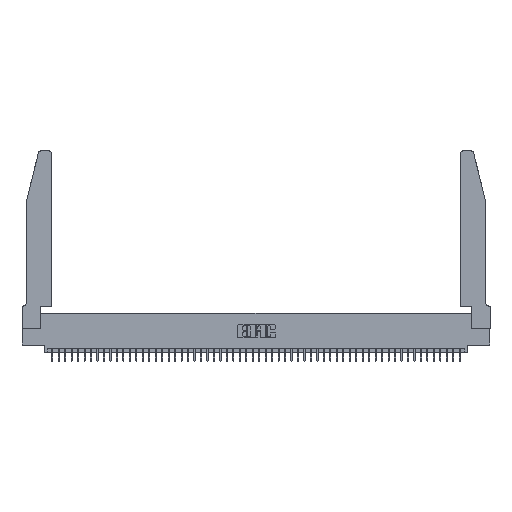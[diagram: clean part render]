
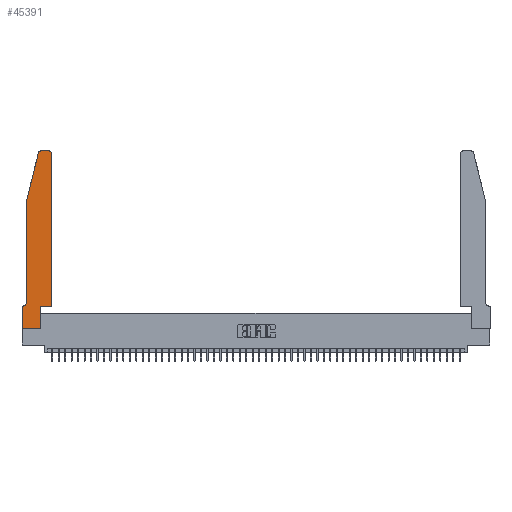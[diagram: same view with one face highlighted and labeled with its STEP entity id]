
A CAD part, top view. The second image highlights one B-rep face of the part: STEP entity #45391.
In plain terms, the highlighted planar face has unit normal (0, 0, 1).
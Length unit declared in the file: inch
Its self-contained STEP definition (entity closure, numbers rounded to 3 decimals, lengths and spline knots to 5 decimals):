
#386 = CARTESIAN_POINT ( 'NONE',  ( 0.284, 2.75, 0.37 ) ) ;
#459 = LINE ( 'NONE', #8402, #41374 ) ;
#460 = ORIENTED_EDGE ( 'NONE', *, *, #44067, .T. ) ;
#944 = CARTESIAN_POINT ( 'NONE',  ( 0.4505, 0.35, 0.37 ) ) ;
#1328 = EDGE_CURVE ( 'NONE', #50639, #6723, #50533, .T. ) ;
#1587 = VERTEX_POINT ( 'NONE', #25113 ) ;
#2338 = AXIS2_PLACEMENT_3D ( 'NONE', #5285, #25363, #17427 ) ;
#2593 = CARTESIAN_POINT ( 'NONE',  ( 0.4205, 2.75, 0.37 ) ) ;
#2871 = LINE ( 'NONE', #31416, #31472 ) ;
#3505 = AXIS2_PLACEMENT_3D ( 'NONE', #18943, #39812, #23174 ) ;
#3706 = ORIENTED_EDGE ( 'NONE', *, *, #1328, .T. ) ;
#4463 = CARTESIAN_POINT ( 'NONE',  ( 0.0055, 0.35, 0.37 ) ) ;
#5285 = CARTESIAN_POINT ( 'NONE',  ( 0.0055, 0.42, 0.37 ) ) ;
#5765 = EDGE_CURVE ( 'NONE', #28128, #6546, #41773, .T. ) ;
#5894 = ORIENTED_EDGE ( 'NONE', *, *, #25072, .T. ) ;
#6160 = AXIS2_PLACEMENT_3D ( 'NONE', #21103, #44902, #8698 ) ;
#6546 = VERTEX_POINT ( 'NONE', #24701 ) ;
#6723 = VERTEX_POINT ( 'NONE', #49540 ) ;
#6933 = ORIENTED_EDGE ( 'NONE', *, *, #7925, .T. ) ;
#7180 = EDGE_CURVE ( 'NONE', #6723, #8515, #17484, .T. ) ;
#7925 = EDGE_CURVE ( 'NONE', #8515, #28151, #41663, .T. ) ;
#8402 = CARTESIAN_POINT ( 'NONE',  ( 0.0755, 2., 0.37 ) ) ;
#8515 = VERTEX_POINT ( 'NONE', #18974 ) ;
#8698 = DIRECTION ( 'NONE',  ( 1., 0., 0. ) ) ;
#10271 = VECTOR ( 'NONE', #13387, 39.37008 ) ;
#11066 = LINE ( 'NONE', #18715, #19585 ) ;
#11080 = DIRECTION ( 'NONE',  ( -1., 0., 0. ) ) ;
#11160 = CARTESIAN_POINT ( 'NONE',  ( 0.0755, 0.42, 0.37 ) ) ;
#12344 = ORIENTED_EDGE ( 'NONE', *, *, #20490, .T. ) ;
#12481 = VECTOR ( 'NONE', #25418, 39.37008 ) ;
#12670 = PLANE ( 'NONE',  #6160 ) ;
#13387 = DIRECTION ( 'NONE',  ( 0., 1., 0. ) ) ;
#14039 = VECTOR ( 'NONE', #21319, 39.37008 ) ;
#14208 = CARTESIAN_POINT ( 'NONE',  ( 0.4505, 0.35, 0.37 ) ) ;
#14576 = DIRECTION ( 'NONE',  ( 1., 0., 0. ) ) ;
#15441 = VERTEX_POINT ( 'NONE', #386 ) ;
#17427 = DIRECTION ( 'NONE',  ( -1., 0., 0. ) ) ;
#17484 = LINE ( 'NONE', #29376, #12481 ) ;
#17785 = VERTEX_POINT ( 'NONE', #25896 ) ;
#18014 = CARTESIAN_POINT ( 'NONE',  ( 0., 0., 0.37 ) ) ;
#18715 = CARTESIAN_POINT ( 'NONE',  ( 0., 0., 0.37 ) ) ;
#18902 = CARTESIAN_POINT ( 'NONE',  ( 0., 0., 0.37 ) ) ;
#18943 = CARTESIAN_POINT ( 'NONE',  ( 0.284, 2.72, 0.37 ) ) ;
#18963 = LINE ( 'NONE', #35858, #27461 ) ;
#18974 = CARTESIAN_POINT ( 'NONE',  ( 0.2865, 0.35, 0.37 ) ) ;
#19585 = VECTOR ( 'NONE', #30608, 39.37008 ) ;
#20490 = EDGE_CURVE ( 'NONE', #37545, #31872, #459, .T. ) ;
#20561 = DIRECTION ( 'NONE',  ( 0., -1., 0. ) ) ;
#21103 = CARTESIAN_POINT ( 'NONE',  ( 0., 0.35, 0.37 ) ) ;
#21319 = DIRECTION ( 'NONE',  ( 1., 0., 0. ) ) ;
#22026 = EDGE_CURVE ( 'NONE', #15441, #1587, #45722, .T. ) ;
#23174 = DIRECTION ( 'NONE',  ( 1., 0., 0. ) ) ;
#23194 = DIRECTION ( 'NONE',  ( -0.239, -0.971, 0. ) ) ;
#24701 = CARTESIAN_POINT ( 'NONE',  ( 0., 0.35, 0.37 ) ) ;
#24888 = ORIENTED_EDGE ( 'NONE', *, *, #36820, .T. ) ;
#25072 = EDGE_CURVE ( 'NONE', #17785, #40887, #40025, .T. ) ;
#25113 = CARTESIAN_POINT ( 'NONE',  ( 0.25487, 2.72718, 0.37 ) ) ;
#25140 = CIRCLE ( 'NONE', #2338, 0.07 ) ;
#25363 = DIRECTION ( 'NONE',  ( 0., 0., -1. ) ) ;
#25418 = DIRECTION ( 'NONE',  ( 0., 1., 0. ) ) ;
#25896 = CARTESIAN_POINT ( 'NONE',  ( 0.4505, 2.72, 0.37 ) ) ;
#26241 = ORIENTED_EDGE ( 'NONE', *, *, #35326, .T. ) ;
#26290 = ORIENTED_EDGE ( 'NONE', *, *, #22026, .T. ) ;
#26847 = DIRECTION ( 'NONE',  ( 0., 0., 1. ) ) ;
#27461 = VECTOR ( 'NONE', #23194, 39.37008 ) ;
#28128 = VERTEX_POINT ( 'NONE', #4463 ) ;
#28151 = VERTEX_POINT ( 'NONE', #14208 ) ;
#29015 = EDGE_CURVE ( 'NONE', #31872, #28128, #25140, .T. ) ;
#29376 = CARTESIAN_POINT ( 'NONE',  ( 0.2865, 0.35, 0.37 ) ) ;
#29507 = VECTOR ( 'NONE', #14576, 39.37008 ) ;
#30608 = DIRECTION ( 'NONE',  ( 0., -1., 0. ) ) ;
#31416 = CARTESIAN_POINT ( 'NONE',  ( 0.2605, 2.75, 0.37 ) ) ;
#31472 = VECTOR ( 'NONE', #11080, 39.37008 ) ;
#31606 = ORIENTED_EDGE ( 'NONE', *, *, #7180, .T. ) ;
#31872 = VERTEX_POINT ( 'NONE', #11160 ) ;
#33075 = DIRECTION ( 'NONE',  ( -1., 0., 0. ) ) ;
#34526 = DIRECTION ( 'NONE',  ( 1., 0., 0. ) ) ;
#34558 = CARTESIAN_POINT ( 'NONE',  ( 0.0755, 2., 0.37 ) ) ;
#35326 = EDGE_CURVE ( 'NONE', #6546, #50639, #11066, .T. ) ;
#35858 = CARTESIAN_POINT ( 'NONE',  ( 0.0755, 2., 0.37 ) ) ;
#36820 = EDGE_CURVE ( 'NONE', #40887, #15441, #2871, .T. ) ;
#37146 = LINE ( 'NONE', #944, #10271 ) ;
#37545 = VERTEX_POINT ( 'NONE', #34558 ) ;
#38294 = AXIS2_PLACEMENT_3D ( 'NONE', #45458, #26847, #34526 ) ;
#39282 = ORIENTED_EDGE ( 'NONE', *, *, #5765, .T. ) ;
#39812 = DIRECTION ( 'NONE',  ( 0., 0., 1. ) ) ;
#40025 = CIRCLE ( 'NONE', #38294, 0.03 ) ;
#40495 = ORIENTED_EDGE ( 'NONE', *, *, #50221, .T. ) ;
#40887 = VERTEX_POINT ( 'NONE', #2593 ) ;
#40891 = CARTESIAN_POINT ( 'NONE',  ( 0.4505, 0.35, 0.37 ) ) ;
#41190 = FACE_OUTER_BOUND ( 'NONE', #44177, .T. ) ;
#41374 = VECTOR ( 'NONE', #20561, 39.37008 ) ;
#41663 = LINE ( 'NONE', #40891, #14039 ) ;
#41773 = LINE ( 'NONE', #44980, #44286 ) ;
#44067 = EDGE_CURVE ( 'NONE', #28151, #17785, #37146, .T. ) ;
#44177 = EDGE_LOOP ( 'NONE', ( #24888, #26290, #40495, #12344, #49740, #39282, #26241, #3706, #31606, #6933, #460, #5894 ) ) ;
#44286 = VECTOR ( 'NONE', #33075, 39.37008 ) ;
#44902 = DIRECTION ( 'NONE',  ( 0., 0., 1. ) ) ;
#44980 = CARTESIAN_POINT ( 'NONE',  ( 0.0755, 0.35, 0.37 ) ) ;
#45391 = ADVANCED_FACE ( 'NONE', ( #41190 ), #12670, .T. ) ;
#45458 = CARTESIAN_POINT ( 'NONE',  ( 0.4205, 2.72, 0.37 ) ) ;
#45722 = CIRCLE ( 'NONE', #3505, 0.03 ) ;
#49540 = CARTESIAN_POINT ( 'NONE',  ( 0.2865, 0., 0.37 ) ) ;
#49740 = ORIENTED_EDGE ( 'NONE', *, *, #29015, .T. ) ;
#50221 = EDGE_CURVE ( 'NONE', #1587, #37545, #18963, .T. ) ;
#50533 = LINE ( 'NONE', #18014, #29507 ) ;
#50639 = VERTEX_POINT ( 'NONE', #18902 ) ;
